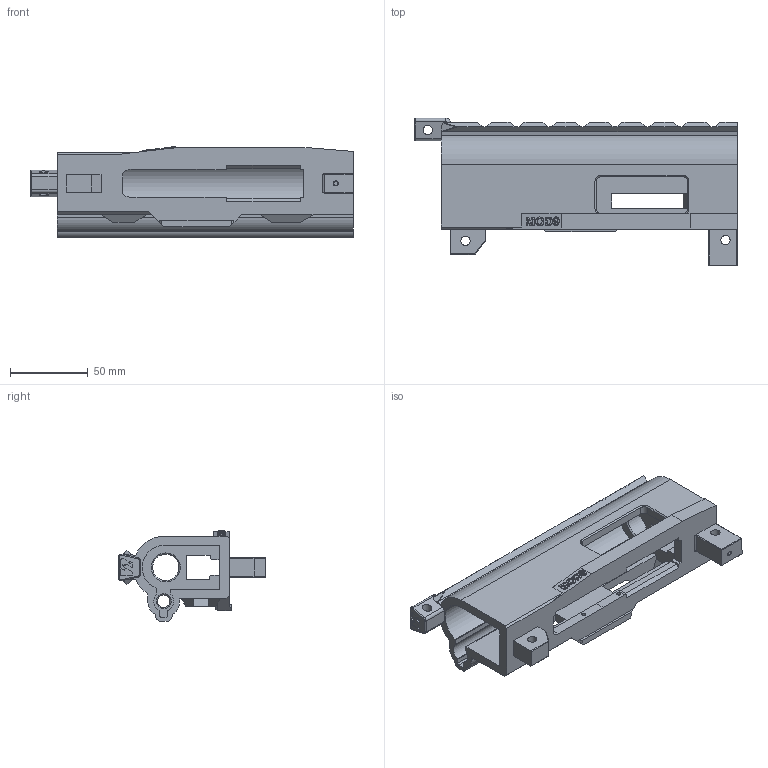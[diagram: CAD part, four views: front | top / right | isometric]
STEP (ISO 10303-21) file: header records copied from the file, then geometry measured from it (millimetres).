
FILE_DESCRIPTION(/* description */ (''),/* implementation_level */ '2;1');
FILE_NAME(/* author */ (''),/* organization */ (''),/* preprocessor_version */ 'ST-DEVELOPER v15.2',/* originating_system */ 'Autodesk Translator Framework v2.0.0.5431',/* authorisation */ '');
FILE_SCHEMA (('AUTOMOTIVE_DESIGN { 1 0 10303 214 3 1 1 }'));
Length unit declared in the file: centimetre
Products named in the file (1): (Unsaved)
Bounding box: 207.36 x 94.9 x 58.41 mm (x, y, z)
Volume: 246654.8 mm3; surface area: 84526.7 mm2
Topology: 1 solids, 2 shells, 511 faces, 1413 edges, 917 vertices
Faces by surface type: plane 265, bspline 156, cylinder 73, cone 13, torus 4
Full cylindrical faces by diameter (mm): 2 x1, 2.4 x4, 2.5 x1, 2.6 x2, 6 x3, 8 x1, 17 x1
Entity records: 19324 total; most frequent: CARTESIAN_POINT 7482, ORIENTED_EDGE 2768, DIRECTION 1859, EDGE_CURVE 1384, VERTEX_POINT 910, LINE 853, VECTOR 853, EDGE_LOOP 568
